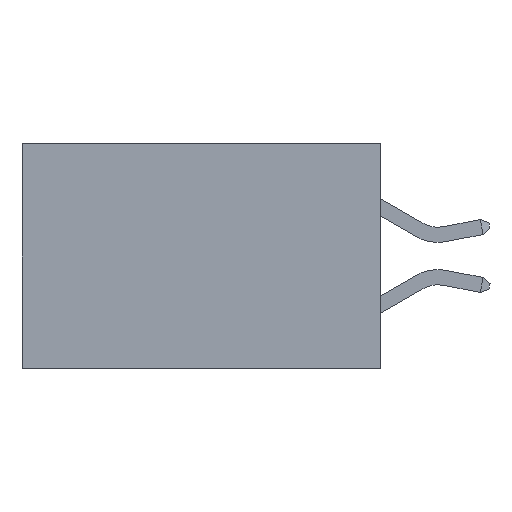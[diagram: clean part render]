
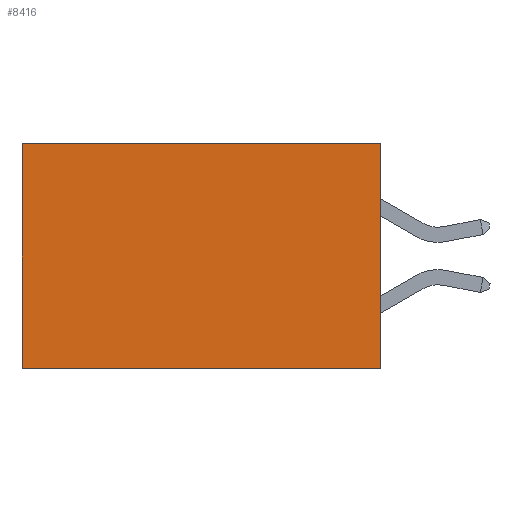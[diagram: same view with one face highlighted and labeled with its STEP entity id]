
A CAD part, left-side view. The second image highlights one B-rep face of the part: STEP entity #8416.
In plain terms, the highlighted planar face has unit normal (-1, 0, 0).
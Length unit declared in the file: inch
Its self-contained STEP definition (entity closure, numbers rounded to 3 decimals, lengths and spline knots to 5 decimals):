
#658 = PLANE ( 'NONE',  #31573 ) ;
#1127 = VERTEX_POINT ( 'NONE', #16944 ) ;
#2190 = CARTESIAN_POINT ( 'NONE',  ( 0.277, 0.59, 0. ) ) ;
#4432 = LINE ( 'NONE', #27163, #18418 ) ;
#4676 = VECTOR ( 'NONE', #25154, 39.37008 ) ;
#5346 = CARTESIAN_POINT ( 'NONE',  ( 0.277, 0., -0.37 ) ) ;
#5812 = VECTOR ( 'NONE', #27759, 39.37008 ) ;
#7476 = ORIENTED_EDGE ( 'NONE', *, *, #23600, .F. ) ;
#8236 = CARTESIAN_POINT ( 'NONE',  ( 0.277, 0., -0.37 ) ) ;
#8416 = ADVANCED_FACE ( 'NONE', ( #15891 ), #658, .F. ) ;
#10533 = CARTESIAN_POINT ( 'NONE',  ( 0.277, 0., 0. ) ) ;
#10763 = DIRECTION ( 'NONE',  ( 1., 0., 0. ) ) ;
#10883 = EDGE_CURVE ( 'NONE', #28838, #14115, #4432, .T. ) ;
#11493 = EDGE_CURVE ( 'NONE', #23442, #1127, #19548, .T. ) ;
#12329 = DIRECTION ( 'NONE',  ( 0., 0., -1. ) ) ;
#13106 = CARTESIAN_POINT ( 'NONE',  ( 0.277, 0., 0. ) ) ;
#14115 = VERTEX_POINT ( 'NONE', #16834 ) ;
#15891 = FACE_OUTER_BOUND ( 'NONE', #20939, .T. ) ;
#16834 = CARTESIAN_POINT ( 'NONE',  ( 0.277, 0., -0.37 ) ) ;
#16944 = CARTESIAN_POINT ( 'NONE',  ( 0.277, 0.59, -0.37 ) ) ;
#17990 = VECTOR ( 'NONE', #31772, 39.37008 ) ;
#18418 = VECTOR ( 'NONE', #12329, 39.37008 ) ;
#19548 = LINE ( 'NONE', #24442, #17990 ) ;
#20638 = ORIENTED_EDGE ( 'NONE', *, *, #11493, .T. ) ;
#20939 = EDGE_LOOP ( 'NONE', ( #20638, #7476, #30071, #26625 ) ) ;
#23442 = VERTEX_POINT ( 'NONE', #2190 ) ;
#23600 = EDGE_CURVE ( 'NONE', #14115, #1127, #30156, .T. ) ;
#24442 = CARTESIAN_POINT ( 'NONE',  ( 0.277, 0.59, -0.37 ) ) ;
#24798 = LINE ( 'NONE', #10533, #5812 ) ;
#25154 = DIRECTION ( 'NONE',  ( 0., 1., 0. ) ) ;
#26100 = EDGE_CURVE ( 'NONE', #28838, #23442, #24798, .T. ) ;
#26625 = ORIENTED_EDGE ( 'NONE', *, *, #26100, .T. ) ;
#27163 = CARTESIAN_POINT ( 'NONE',  ( 0.277, 0., -0.37 ) ) ;
#27759 = DIRECTION ( 'NONE',  ( 0., 1., 0. ) ) ;
#27988 = DIRECTION ( 'NONE',  ( 0., 0., -1. ) ) ;
#28838 = VERTEX_POINT ( 'NONE', #13106 ) ;
#30071 = ORIENTED_EDGE ( 'NONE', *, *, #10883, .F. ) ;
#30156 = LINE ( 'NONE', #5346, #4676 ) ;
#31573 = AXIS2_PLACEMENT_3D ( 'NONE', #8236, #10763, #27988 ) ;
#31772 = DIRECTION ( 'NONE',  ( 0., 0., -1. ) ) ;
